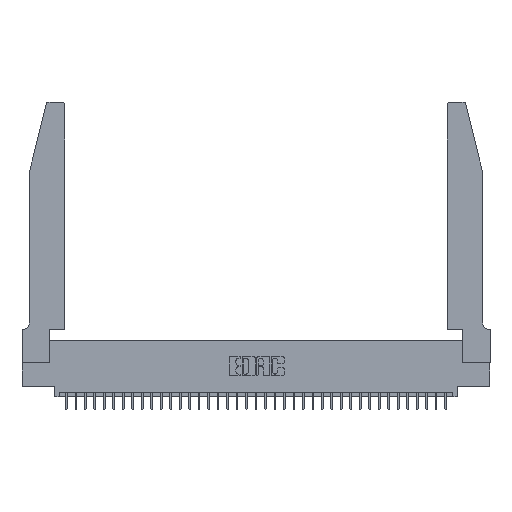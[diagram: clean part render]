
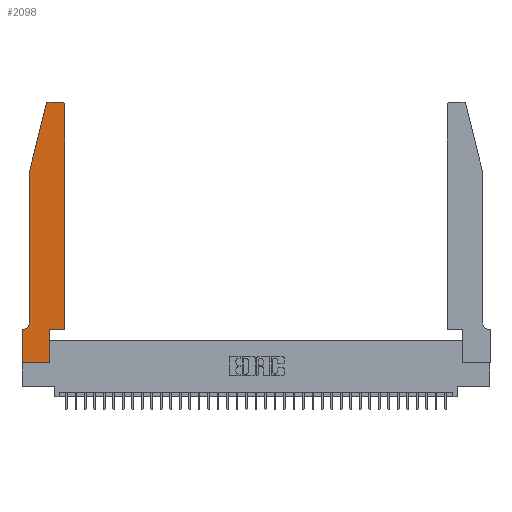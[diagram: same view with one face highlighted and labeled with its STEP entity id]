
A CAD part, top view. The second image highlights one B-rep face of the part: STEP entity #2098.
In plain terms, the highlighted planar face has unit normal (0, 0, 1).
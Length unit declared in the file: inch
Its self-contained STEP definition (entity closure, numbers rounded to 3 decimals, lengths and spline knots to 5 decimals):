
#2048 = EDGE_CURVE ( 'NONE', #20774, #21993, #25836, .T. ) ;
#2098 = ADVANCED_FACE ( 'NONE', ( #3365 ), #12406, .T. ) ;
#2121 = ORIENTED_EDGE ( 'NONE', *, *, #16405, .T. ) ;
#2145 = ORIENTED_EDGE ( 'NONE', *, *, #33946, .T. ) ;
#2237 = CARTESIAN_POINT ( 'NONE',  ( 0.2865, 0.35, 0.37 ) ) ;
#2358 = DIRECTION ( 'NONE',  ( -1., 0., 0. ) ) ;
#2616 = DIRECTION ( 'NONE',  ( -0.239, -0.971, 0. ) ) ;
#2765 = AXIS2_PLACEMENT_3D ( 'NONE', #36006, #15224, #7277 ) ;
#3003 = ORIENTED_EDGE ( 'NONE', *, *, #11105, .T. ) ;
#3365 = FACE_OUTER_BOUND ( 'NONE', #33205, .T. ) ;
#3393 = ORIENTED_EDGE ( 'NONE', *, *, #15784, .T. ) ;
#3547 = VECTOR ( 'NONE', #8976, 39.37008 ) ;
#3785 = VECTOR ( 'NONE', #29527, 39.37008 ) ;
#4148 = CARTESIAN_POINT ( 'NONE',  ( 0.284, 2.72, 0.37 ) ) ;
#4334 = DIRECTION ( 'NONE',  ( 0., 0., 1. ) ) ;
#4352 = EDGE_CURVE ( 'NONE', #18386, #24040, #37240, .T. ) ;
#4951 = DIRECTION ( 'NONE',  ( 1., 0., 0. ) ) ;
#5537 = CARTESIAN_POINT ( 'NONE',  ( 0.0755, 0.35, 0.37 ) ) ;
#6952 = VERTEX_POINT ( 'NONE', #29804 ) ;
#7277 = DIRECTION ( 'NONE',  ( 1., 0., 0. ) ) ;
#7728 = EDGE_CURVE ( 'NONE', #15962, #23571, #7777, .T. ) ;
#7777 = LINE ( 'NONE', #33861, #12783 ) ;
#8284 = AXIS2_PLACEMENT_3D ( 'NONE', #28730, #31218, #26093 ) ;
#8976 = DIRECTION ( 'NONE',  ( 0., -1., 0. ) ) ;
#9360 = LINE ( 'NONE', #23872, #3547 ) ;
#10105 = LINE ( 'NONE', #26928, #11774 ) ;
#10295 = VERTEX_POINT ( 'NONE', #13214 ) ;
#10372 = VECTOR ( 'NONE', #22430, 39.37008 ) ;
#10559 = CARTESIAN_POINT ( 'NONE',  ( 0.0755, 2., 0.37 ) ) ;
#10738 = LINE ( 'NONE', #10559, #16011 ) ;
#10893 = LINE ( 'NONE', #2237, #10372 ) ;
#10970 = CIRCLE ( 'NONE', #21857, 0.03 ) ;
#11105 = EDGE_CURVE ( 'NONE', #24040, #20891, #14049, .T. ) ;
#11774 = VECTOR ( 'NONE', #30146, 39.37008 ) ;
#12213 = CARTESIAN_POINT ( 'NONE',  ( 0., 0.35, 0.37 ) ) ;
#12406 = PLANE ( 'NONE',  #17553 ) ;
#12733 = VERTEX_POINT ( 'NONE', #33733 ) ;
#12783 = VECTOR ( 'NONE', #4951, 39.37008 ) ;
#13214 = CARTESIAN_POINT ( 'NONE',  ( 0.4505, 2.72, 0.37 ) ) ;
#14049 = LINE ( 'NONE', #5537, #18086 ) ;
#14802 = ORIENTED_EDGE ( 'NONE', *, *, #4352, .T. ) ;
#15138 = CARTESIAN_POINT ( 'NONE',  ( 0.2865, 0., 0.37 ) ) ;
#15224 = DIRECTION ( 'NONE',  ( 0., 0., 1. ) ) ;
#15784 = EDGE_CURVE ( 'NONE', #21993, #18386, #10738, .T. ) ;
#15951 = CARTESIAN_POINT ( 'NONE',  ( 0.4505, 0.35, 0.37 ) ) ;
#15962 = VERTEX_POINT ( 'NONE', #21676 ) ;
#16011 = VECTOR ( 'NONE', #24928, 39.37008 ) ;
#16405 = EDGE_CURVE ( 'NONE', #12733, #30140, #10105, .T. ) ;
#16565 = EDGE_CURVE ( 'NONE', #10295, #12733, #34759, .T. ) ;
#17064 = ORIENTED_EDGE ( 'NONE', *, *, #16565, .T. ) ;
#17553 = AXIS2_PLACEMENT_3D ( 'NONE', #12213, #34909, #20526 ) ;
#18086 = VECTOR ( 'NONE', #2358, 39.37008 ) ;
#18272 = ORIENTED_EDGE ( 'NONE', *, *, #18609, .T. ) ;
#18300 = DIRECTION ( 'NONE',  ( 1., 0., 0. ) ) ;
#18386 = VERTEX_POINT ( 'NONE', #23945 ) ;
#18609 = EDGE_CURVE ( 'NONE', #23571, #6952, #10893, .T. ) ;
#19367 = EDGE_CURVE ( 'NONE', #6952, #24589, #32203, .T. ) ;
#19986 = CARTESIAN_POINT ( 'NONE',  ( 0.0055, 0.35, 0.37 ) ) ;
#20256 = CARTESIAN_POINT ( 'NONE',  ( 0.4505, 0.35, 0.37 ) ) ;
#20526 = DIRECTION ( 'NONE',  ( 1., 0., 0. ) ) ;
#20774 = VERTEX_POINT ( 'NONE', #35790 ) ;
#20891 = VERTEX_POINT ( 'NONE', #22875 ) ;
#21619 = VECTOR ( 'NONE', #27477, 39.37008 ) ;
#21676 = CARTESIAN_POINT ( 'NONE',  ( 0., 0., 0.37 ) ) ;
#21857 = AXIS2_PLACEMENT_3D ( 'NONE', #4148, #4334, #18300 ) ;
#21993 = VERTEX_POINT ( 'NONE', #29030 ) ;
#22430 = DIRECTION ( 'NONE',  ( 0., 1., 0. ) ) ;
#22875 = CARTESIAN_POINT ( 'NONE',  ( 0., 0.35, 0.37 ) ) ;
#22984 = CARTESIAN_POINT ( 'NONE',  ( 0.0755, 2., 0.37 ) ) ;
#23331 = ORIENTED_EDGE ( 'NONE', *, *, #19367, .T. ) ;
#23571 = VERTEX_POINT ( 'NONE', #15138 ) ;
#23872 = CARTESIAN_POINT ( 'NONE',  ( 0., 0., 0.37 ) ) ;
#23945 = CARTESIAN_POINT ( 'NONE',  ( 0.0755, 0.42, 0.37 ) ) ;
#24040 = VERTEX_POINT ( 'NONE', #19986 ) ;
#24208 = EDGE_CURVE ( 'NONE', #30140, #20774, #10970, .T. ) ;
#24209 = ORIENTED_EDGE ( 'NONE', *, *, #2048, .T. ) ;
#24589 = VERTEX_POINT ( 'NONE', #35087 ) ;
#24690 = CARTESIAN_POINT ( 'NONE',  ( 0.284, 2.75, 0.37 ) ) ;
#24720 = ORIENTED_EDGE ( 'NONE', *, *, #24208, .T. ) ;
#24928 = DIRECTION ( 'NONE',  ( 0., -1., 0. ) ) ;
#25836 = LINE ( 'NONE', #22984, #35706 ) ;
#26093 = DIRECTION ( 'NONE',  ( -1., 0., 0. ) ) ;
#26928 = CARTESIAN_POINT ( 'NONE',  ( 0.2605, 2.75, 0.37 ) ) ;
#27109 = LINE ( 'NONE', #15951, #21619 ) ;
#27377 = ORIENTED_EDGE ( 'NONE', *, *, #34054, .T. ) ;
#27477 = DIRECTION ( 'NONE',  ( 0., 1., 0. ) ) ;
#28730 = CARTESIAN_POINT ( 'NONE',  ( 0.0055, 0.42, 0.37 ) ) ;
#29030 = CARTESIAN_POINT ( 'NONE',  ( 0.0755, 2., 0.37 ) ) ;
#29527 = DIRECTION ( 'NONE',  ( 1., 0., 0. ) ) ;
#29804 = CARTESIAN_POINT ( 'NONE',  ( 0.2865, 0.35, 0.37 ) ) ;
#30140 = VERTEX_POINT ( 'NONE', #24690 ) ;
#30146 = DIRECTION ( 'NONE',  ( -1., 0., 0. ) ) ;
#31218 = DIRECTION ( 'NONE',  ( 0., 0., -1. ) ) ;
#31659 = ORIENTED_EDGE ( 'NONE', *, *, #7728, .T. ) ;
#32203 = LINE ( 'NONE', #20256, #3785 ) ;
#33205 = EDGE_LOOP ( 'NONE', ( #2121, #24720, #24209, #3393, #14802, #3003, #2145, #31659, #18272, #23331, #27377, #17064 ) ) ;
#33733 = CARTESIAN_POINT ( 'NONE',  ( 0.4205, 2.75, 0.37 ) ) ;
#33861 = CARTESIAN_POINT ( 'NONE',  ( 0., 0., 0.37 ) ) ;
#33946 = EDGE_CURVE ( 'NONE', #20891, #15962, #9360, .T. ) ;
#34054 = EDGE_CURVE ( 'NONE', #24589, #10295, #27109, .T. ) ;
#34759 = CIRCLE ( 'NONE', #2765, 0.03 ) ;
#34909 = DIRECTION ( 'NONE',  ( 0., 0., 1. ) ) ;
#35087 = CARTESIAN_POINT ( 'NONE',  ( 0.4505, 0.35, 0.37 ) ) ;
#35706 = VECTOR ( 'NONE', #2616, 39.37008 ) ;
#35790 = CARTESIAN_POINT ( 'NONE',  ( 0.25487, 2.72718, 0.37 ) ) ;
#36006 = CARTESIAN_POINT ( 'NONE',  ( 0.4205, 2.72, 0.37 ) ) ;
#37240 = CIRCLE ( 'NONE', #8284, 0.07 ) ;
